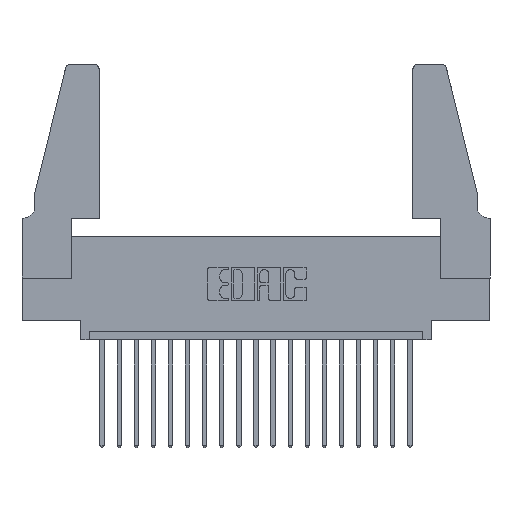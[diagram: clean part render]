
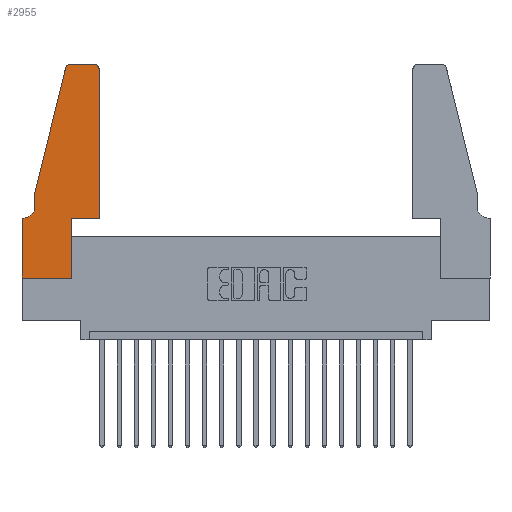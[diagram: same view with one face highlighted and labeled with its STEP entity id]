
A CAD part, top view. The second image highlights one B-rep face of the part: STEP entity #2955.
In plain terms, the highlighted planar face has unit normal (0, 0, 1).
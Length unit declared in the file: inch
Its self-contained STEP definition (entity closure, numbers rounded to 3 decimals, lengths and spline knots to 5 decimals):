
#149 = CARTESIAN_POINT ( 'NONE',  ( 0.25487, 1.22718, 0.37 ) ) ;
#205 = VECTOR ( 'NONE', #15483, 39.37008 ) ;
#964 = LINE ( 'NONE', #3817, #9113 ) ;
#1004 = EDGE_CURVE ( 'NONE', #17570, #14381, #7726, .T. ) ;
#1210 = CARTESIAN_POINT ( 'NONE',  ( 0.4505, 0.35, 0.37 ) ) ;
#1404 = DIRECTION ( 'NONE',  ( 0., 0., -1. ) ) ;
#1680 = VECTOR ( 'NONE', #4887, 39.37008 ) ;
#1695 = CIRCLE ( 'NONE', #8150, 0.03 ) ;
#1802 = CARTESIAN_POINT ( 'NONE',  ( 0.2605, 1.25, 0.37 ) ) ;
#1929 = ORIENTED_EDGE ( 'NONE', *, *, #8763, .T. ) ;
#1958 = ORIENTED_EDGE ( 'NONE', *, *, #16641, .T. ) ;
#2106 = LINE ( 'NONE', #1210, #18044 ) ;
#2213 = CARTESIAN_POINT ( 'NONE',  ( 0., 0., 0.37 ) ) ;
#2228 = VECTOR ( 'NONE', #7500, 39.37008 ) ;
#2339 = CARTESIAN_POINT ( 'NONE',  ( 0., 0., 0.37 ) ) ;
#2376 = CARTESIAN_POINT ( 'NONE',  ( 0., 0.35, 0.37 ) ) ;
#2513 = EDGE_CURVE ( 'NONE', #9409, #17570, #18011, .T. ) ;
#2694 = DIRECTION ( 'NONE',  ( 1., 0., 0. ) ) ;
#2955 = ADVANCED_FACE ( 'NONE', ( #11392 ), #11476, .T. ) ;
#3817 = CARTESIAN_POINT ( 'NONE',  ( 0.0755, 0.5, 0.37 ) ) ;
#3818 = LINE ( 'NONE', #10216, #205 ) ;
#3910 = DIRECTION ( 'NONE',  ( 0., -1., 0. ) ) ;
#3996 = AXIS2_PLACEMENT_3D ( 'NONE', #13541, #1404, #14976 ) ;
#4012 = CARTESIAN_POINT ( 'NONE',  ( 0.284, 1.25, 0.37 ) ) ;
#4153 = ORIENTED_EDGE ( 'NONE', *, *, #10747, .T. ) ;
#4513 = AXIS2_PLACEMENT_3D ( 'NONE', #2376, #13069, #14509 ) ;
#4644 = CARTESIAN_POINT ( 'NONE',  ( 0.2865, 0., 0.37 ) ) ;
#4872 = DIRECTION ( 'NONE',  ( 0., 1., 0. ) ) ;
#4887 = DIRECTION ( 'NONE',  ( -1., 0., 0. ) ) ;
#5022 = DIRECTION ( 'NONE',  ( 1., 0., 0. ) ) ;
#5027 = CARTESIAN_POINT ( 'NONE',  ( 0.2865, 0.35, 0.37 ) ) ;
#5185 = VERTEX_POINT ( 'NONE', #149 ) ;
#5220 = CARTESIAN_POINT ( 'NONE',  ( 0.0755, 0.5, 0.37 ) ) ;
#5618 = LINE ( 'NONE', #7787, #11141 ) ;
#5963 = VECTOR ( 'NONE', #11914, 39.37008 ) ;
#6061 = EDGE_CURVE ( 'NONE', #7349, #12237, #13603, .T. ) ;
#6603 = CARTESIAN_POINT ( 'NONE',  ( 0.4505, 1.22, 0.37 ) ) ;
#6690 = ORIENTED_EDGE ( 'NONE', *, *, #2513, .T. ) ;
#6924 = LINE ( 'NONE', #1802, #1680 ) ;
#7089 = VERTEX_POINT ( 'NONE', #4644 ) ;
#7197 = LINE ( 'NONE', #2339, #10077 ) ;
#7349 = VERTEX_POINT ( 'NONE', #13066 ) ;
#7500 = DIRECTION ( 'NONE',  ( -1., 0., 0. ) ) ;
#7726 = LINE ( 'NONE', #10655, #2228 ) ;
#7787 = CARTESIAN_POINT ( 'NONE',  ( 0.2865, 0.35, 0.37 ) ) ;
#8047 = VERTEX_POINT ( 'NONE', #15654 ) ;
#8150 = AXIS2_PLACEMENT_3D ( 'NONE', #16163, #17669, #10161 ) ;
#8763 = EDGE_CURVE ( 'NONE', #14910, #9409, #12716, .T. ) ;
#9113 = VECTOR ( 'NONE', #11848, 39.37008 ) ;
#9409 = VERTEX_POINT ( 'NONE', #18688 ) ;
#9593 = CIRCLE ( 'NONE', #17280, 0.03 ) ;
#9689 = DIRECTION ( 'NONE',  ( 0., -1., 0. ) ) ;
#10077 = VECTOR ( 'NONE', #3910, 39.37008 ) ;
#10161 = DIRECTION ( 'NONE',  ( 1., 0., 0. ) ) ;
#10193 = ORIENTED_EDGE ( 'NONE', *, *, #14998, .T. ) ;
#10216 = CARTESIAN_POINT ( 'NONE',  ( 0., 0., 0.37 ) ) ;
#10381 = CARTESIAN_POINT ( 'NONE',  ( 0.0055, 0.35, 0.37 ) ) ;
#10462 = EDGE_CURVE ( 'NONE', #12237, #8047, #1695, .T. ) ;
#10655 = CARTESIAN_POINT ( 'NONE',  ( 0.0755, 0.35, 0.37 ) ) ;
#10747 = EDGE_CURVE ( 'NONE', #16465, #5185, #9593, .T. ) ;
#11069 = EDGE_CURVE ( 'NONE', #8047, #16465, #6924, .T. ) ;
#11141 = VECTOR ( 'NONE', #4872, 39.37008 ) ;
#11319 = ORIENTED_EDGE ( 'NONE', *, *, #11069, .T. ) ;
#11392 = FACE_OUTER_BOUND ( 'NONE', #19658, .T. ) ;
#11476 = PLANE ( 'NONE',  #4513 ) ;
#11848 = DIRECTION ( 'NONE',  ( -0.239, -0.971, 0. ) ) ;
#11914 = DIRECTION ( 'NONE',  ( 0., 1., 0. ) ) ;
#12225 = VECTOR ( 'NONE', #9689, 39.37008 ) ;
#12237 = VERTEX_POINT ( 'NONE', #6603 ) ;
#12548 = DIRECTION ( 'NONE',  ( 0., 0., 1. ) ) ;
#12646 = ORIENTED_EDGE ( 'NONE', *, *, #6061, .T. ) ;
#12716 = LINE ( 'NONE', #15753, #12225 ) ;
#12821 = ORIENTED_EDGE ( 'NONE', *, *, #1004, .T. ) ;
#13066 = CARTESIAN_POINT ( 'NONE',  ( 0.4505, 0.35, 0.37 ) ) ;
#13069 = DIRECTION ( 'NONE',  ( 0., 0., 1. ) ) ;
#13541 = CARTESIAN_POINT ( 'NONE',  ( 0.0055, 0.42, 0.37 ) ) ;
#13603 = LINE ( 'NONE', #16594, #5963 ) ;
#14003 = ORIENTED_EDGE ( 'NONE', *, *, #17343, .T. ) ;
#14381 = VERTEX_POINT ( 'NONE', #15976 ) ;
#14410 = ORIENTED_EDGE ( 'NONE', *, *, #10462, .T. ) ;
#14509 = DIRECTION ( 'NONE',  ( 1., 0., 0. ) ) ;
#14910 = VERTEX_POINT ( 'NONE', #5220 ) ;
#14976 = DIRECTION ( 'NONE',  ( -1., 0., 0. ) ) ;
#14998 = EDGE_CURVE ( 'NONE', #14381, #19575, #7197, .T. ) ;
#15355 = EDGE_CURVE ( 'NONE', #5185, #14910, #964, .T. ) ;
#15483 = DIRECTION ( 'NONE',  ( 1., 0., 0. ) ) ;
#15654 = CARTESIAN_POINT ( 'NONE',  ( 0.4205, 1.25, 0.37 ) ) ;
#15753 = CARTESIAN_POINT ( 'NONE',  ( 0.0755, 0.5, 0.37 ) ) ;
#15976 = CARTESIAN_POINT ( 'NONE',  ( 0., 0.35, 0.37 ) ) ;
#16163 = CARTESIAN_POINT ( 'NONE',  ( 0.4205, 1.22, 0.37 ) ) ;
#16465 = VERTEX_POINT ( 'NONE', #4012 ) ;
#16594 = CARTESIAN_POINT ( 'NONE',  ( 0.4505, 0.35, 0.37 ) ) ;
#16641 = EDGE_CURVE ( 'NONE', #17064, #7349, #2106, .T. ) ;
#17064 = VERTEX_POINT ( 'NONE', #5027 ) ;
#17076 = CARTESIAN_POINT ( 'NONE',  ( 0.284, 1.22, 0.37 ) ) ;
#17280 = AXIS2_PLACEMENT_3D ( 'NONE', #17076, #12548, #5022 ) ;
#17343 = EDGE_CURVE ( 'NONE', #19575, #7089, #3818, .T. ) ;
#17570 = VERTEX_POINT ( 'NONE', #10381 ) ;
#17669 = DIRECTION ( 'NONE',  ( 0., 0., 1. ) ) ;
#18011 = CIRCLE ( 'NONE', #3996, 0.07 ) ;
#18044 = VECTOR ( 'NONE', #2694, 39.37008 ) ;
#18688 = CARTESIAN_POINT ( 'NONE',  ( 0.0755, 0.42, 0.37 ) ) ;
#18853 = EDGE_CURVE ( 'NONE', #7089, #17064, #5618, .T. ) ;
#18960 = ORIENTED_EDGE ( 'NONE', *, *, #15355, .T. ) ;
#19041 = ORIENTED_EDGE ( 'NONE', *, *, #18853, .T. ) ;
#19575 = VERTEX_POINT ( 'NONE', #2213 ) ;
#19658 = EDGE_LOOP ( 'NONE', ( #11319, #4153, #18960, #1929, #6690, #12821, #10193, #14003, #19041, #1958, #12646, #14410 ) ) ;
